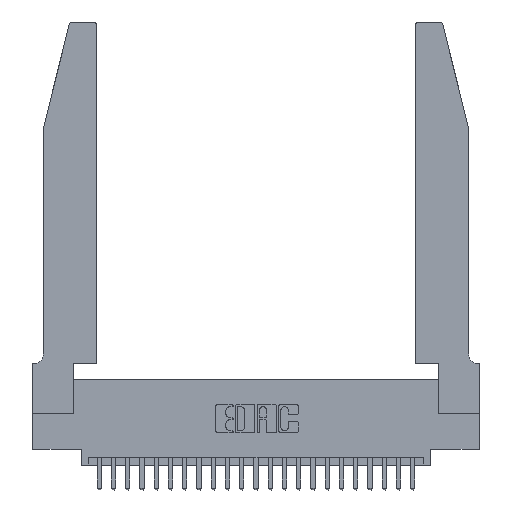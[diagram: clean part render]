
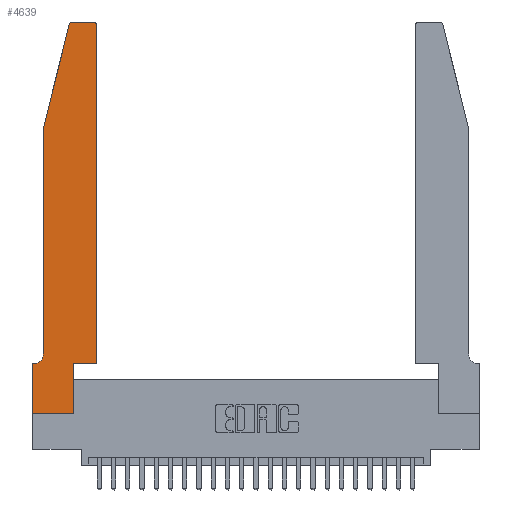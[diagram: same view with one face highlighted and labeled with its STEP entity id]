
A CAD part, top view. The second image highlights one B-rep face of the part: STEP entity #4639.
In plain terms, the highlighted planar face has unit normal (0, 0, 1).
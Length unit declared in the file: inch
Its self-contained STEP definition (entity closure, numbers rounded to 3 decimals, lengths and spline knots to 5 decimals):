
#401 = LINE ( 'NONE', #13441, #4560 ) ;
#584 = ORIENTED_EDGE ( 'NONE', *, *, #3608, .T. ) ;
#788 = VERTEX_POINT ( 'NONE', #7813 ) ;
#928 = DIRECTION ( 'NONE',  ( 1., 0., 0. ) ) ;
#1090 = VERTEX_POINT ( 'NONE', #2482 ) ;
#1208 = DIRECTION ( 'NONE',  ( 0., -1., 0. ) ) ;
#1362 = EDGE_CURVE ( 'NONE', #19335, #11424, #12665, .T. ) ;
#1983 = CARTESIAN_POINT ( 'NONE',  ( 0.0755, 0.35, 0.37 ) ) ;
#2372 = VERTEX_POINT ( 'NONE', #9589 ) ;
#2482 = CARTESIAN_POINT ( 'NONE',  ( 0.25487, 2.72718, 0.37 ) ) ;
#3075 = VERTEX_POINT ( 'NONE', #18757 ) ;
#3132 = VERTEX_POINT ( 'NONE', #16886 ) ;
#3309 = AXIS2_PLACEMENT_3D ( 'NONE', #6061, #19885, #8079 ) ;
#3319 = CARTESIAN_POINT ( 'NONE',  ( 0., 0., 0.37 ) ) ;
#3353 = LINE ( 'NONE', #1983, #23688 ) ;
#3606 = ORIENTED_EDGE ( 'NONE', *, *, #20388, .T. ) ;
#3608 = EDGE_CURVE ( 'NONE', #25214, #14380, #3353, .T. ) ;
#4036 = ORIENTED_EDGE ( 'NONE', *, *, #24233, .T. ) ;
#4391 = DIRECTION ( 'NONE',  ( -1., 0., 0. ) ) ;
#4560 = VECTOR ( 'NONE', #15399, 39.37008 ) ;
#4639 = ADVANCED_FACE ( 'NONE', ( #18807 ), #21670, .T. ) ;
#4955 = DIRECTION ( 'NONE',  ( 0., 1., 0. ) ) ;
#5548 = ORIENTED_EDGE ( 'NONE', *, *, #7864, .T. ) ;
#5849 = CARTESIAN_POINT ( 'NONE',  ( 0.4205, 2.72, 0.37 ) ) ;
#6061 = CARTESIAN_POINT ( 'NONE',  ( 0.0055, 0.42, 0.37 ) ) ;
#6112 = LINE ( 'NONE', #21048, #10882 ) ;
#7813 = CARTESIAN_POINT ( 'NONE',  ( 0.4205, 2.75, 0.37 ) ) ;
#7860 = DIRECTION ( 'NONE',  ( 1., 0., 0. ) ) ;
#7864 = EDGE_CURVE ( 'NONE', #14380, #21037, #22601, .T. ) ;
#8076 = CARTESIAN_POINT ( 'NONE',  ( 0., 0., 0.37 ) ) ;
#8079 = DIRECTION ( 'NONE',  ( -1., 0., 0. ) ) ;
#8323 = EDGE_LOOP ( 'NONE', ( #3606, #19702, #20707, #24893, #4036, #584, #5548, #25027, #17036, #14702, #10532, #9103 ) ) ;
#9103 = ORIENTED_EDGE ( 'NONE', *, *, #11333, .T. ) ;
#9249 = EDGE_CURVE ( 'NONE', #10340, #19335, #18611, .T. ) ;
#9484 = CARTESIAN_POINT ( 'NONE',  ( 0.284, 2.75, 0.37 ) ) ;
#9589 = CARTESIAN_POINT ( 'NONE',  ( 0.2865, 0., 0.37 ) ) ;
#9789 = DIRECTION ( 'NONE',  ( -0.239, -0.971, 0. ) ) ;
#9977 = DIRECTION ( 'NONE',  ( 0., 0., 1. ) ) ;
#10340 = VERTEX_POINT ( 'NONE', #14722 ) ;
#10532 = ORIENTED_EDGE ( 'NONE', *, *, #1362, .T. ) ;
#10882 = VECTOR ( 'NONE', #1208, 39.37008 ) ;
#11009 = CIRCLE ( 'NONE', #17827, 0.03 ) ;
#11070 = EDGE_CURVE ( 'NONE', #15478, #1090, #11009, .T. ) ;
#11333 = EDGE_CURVE ( 'NONE', #11424, #788, #15903, .T. ) ;
#11424 = VERTEX_POINT ( 'NONE', #23694 ) ;
#11457 = CARTESIAN_POINT ( 'NONE',  ( 0., 0., 0.37 ) ) ;
#11460 = DIRECTION ( 'NONE',  ( 0., -1., 0. ) ) ;
#12050 = VECTOR ( 'NONE', #14383, 39.37008 ) ;
#12665 = LINE ( 'NONE', #15515, #12050 ) ;
#13076 = EDGE_CURVE ( 'NONE', #1090, #3075, #19439, .T. ) ;
#13077 = DIRECTION ( 'NONE',  ( 0., 0., 1. ) ) ;
#13367 = LINE ( 'NONE', #16865, #23643 ) ;
#13441 = CARTESIAN_POINT ( 'NONE',  ( 0.2605, 2.75, 0.37 ) ) ;
#13473 = VECTOR ( 'NONE', #23073, 39.37008 ) ;
#13531 = AXIS2_PLACEMENT_3D ( 'NONE', #15846, #9977, #23586 ) ;
#13790 = CARTESIAN_POINT ( 'NONE',  ( 0.0755, 2., 0.37 ) ) ;
#14045 = EDGE_CURVE ( 'NONE', #2372, #10340, #13367, .T. ) ;
#14380 = VERTEX_POINT ( 'NONE', #25538 ) ;
#14383 = DIRECTION ( 'NONE',  ( 0., 1., 0. ) ) ;
#14702 = ORIENTED_EDGE ( 'NONE', *, *, #9249, .T. ) ;
#14722 = CARTESIAN_POINT ( 'NONE',  ( 0.2865, 0.35, 0.37 ) ) ;
#15399 = DIRECTION ( 'NONE',  ( -1., 0., 0. ) ) ;
#15478 = VERTEX_POINT ( 'NONE', #9484 ) ;
#15515 = CARTESIAN_POINT ( 'NONE',  ( 0.4505, 0.35, 0.37 ) ) ;
#15846 = CARTESIAN_POINT ( 'NONE',  ( 0., 0.35, 0.37 ) ) ;
#15903 = CIRCLE ( 'NONE', #18632, 0.03 ) ;
#16021 = EDGE_CURVE ( 'NONE', #21037, #2372, #23222, .T. ) ;
#16756 = CARTESIAN_POINT ( 'NONE',  ( 0.0055, 0.35, 0.37 ) ) ;
#16865 = CARTESIAN_POINT ( 'NONE',  ( 0.2865, 0.35, 0.37 ) ) ;
#16886 = CARTESIAN_POINT ( 'NONE',  ( 0.0755, 0.42, 0.37 ) ) ;
#17036 = ORIENTED_EDGE ( 'NONE', *, *, #14045, .T. ) ;
#17803 = CARTESIAN_POINT ( 'NONE',  ( 0.4505, 0.35, 0.37 ) ) ;
#17827 = AXIS2_PLACEMENT_3D ( 'NONE', #24630, #13077, #928 ) ;
#18611 = LINE ( 'NONE', #19210, #13473 ) ;
#18632 = AXIS2_PLACEMENT_3D ( 'NONE', #5849, #19668, #7860 ) ;
#18757 = CARTESIAN_POINT ( 'NONE',  ( 0.0755, 2., 0.37 ) ) ;
#18807 = FACE_OUTER_BOUND ( 'NONE', #8323, .T. ) ;
#19210 = CARTESIAN_POINT ( 'NONE',  ( 0.4505, 0.35, 0.37 ) ) ;
#19335 = VERTEX_POINT ( 'NONE', #17803 ) ;
#19439 = LINE ( 'NONE', #13790, #24539 ) ;
#19668 = DIRECTION ( 'NONE',  ( 0., 0., 1. ) ) ;
#19702 = ORIENTED_EDGE ( 'NONE', *, *, #11070, .T. ) ;
#19885 = DIRECTION ( 'NONE',  ( 0., 0., -1. ) ) ;
#19922 = VECTOR ( 'NONE', #21821, 39.37008 ) ;
#20388 = EDGE_CURVE ( 'NONE', #788, #15478, #401, .T. ) ;
#20707 = ORIENTED_EDGE ( 'NONE', *, *, #13076, .T. ) ;
#21009 = EDGE_CURVE ( 'NONE', #3075, #3132, #6112, .T. ) ;
#21037 = VERTEX_POINT ( 'NONE', #11457 ) ;
#21048 = CARTESIAN_POINT ( 'NONE',  ( 0.0755, 2., 0.37 ) ) ;
#21186 = CIRCLE ( 'NONE', #3309, 0.07 ) ;
#21670 = PLANE ( 'NONE',  #13531 ) ;
#21821 = DIRECTION ( 'NONE',  ( 1., 0., 0. ) ) ;
#22000 = VECTOR ( 'NONE', #11460, 39.37008 ) ;
#22601 = LINE ( 'NONE', #3319, #22000 ) ;
#23073 = DIRECTION ( 'NONE',  ( 1., 0., 0. ) ) ;
#23222 = LINE ( 'NONE', #8076, #19922 ) ;
#23586 = DIRECTION ( 'NONE',  ( 1., 0., 0. ) ) ;
#23643 = VECTOR ( 'NONE', #4955, 39.37008 ) ;
#23688 = VECTOR ( 'NONE', #4391, 39.37008 ) ;
#23694 = CARTESIAN_POINT ( 'NONE',  ( 0.4505, 2.72, 0.37 ) ) ;
#24233 = EDGE_CURVE ( 'NONE', #3132, #25214, #21186, .T. ) ;
#24539 = VECTOR ( 'NONE', #9789, 39.37008 ) ;
#24630 = CARTESIAN_POINT ( 'NONE',  ( 0.284, 2.72, 0.37 ) ) ;
#24893 = ORIENTED_EDGE ( 'NONE', *, *, #21009, .T. ) ;
#25027 = ORIENTED_EDGE ( 'NONE', *, *, #16021, .T. ) ;
#25214 = VERTEX_POINT ( 'NONE', #16756 ) ;
#25538 = CARTESIAN_POINT ( 'NONE',  ( 0., 0.35, 0.37 ) ) ;
